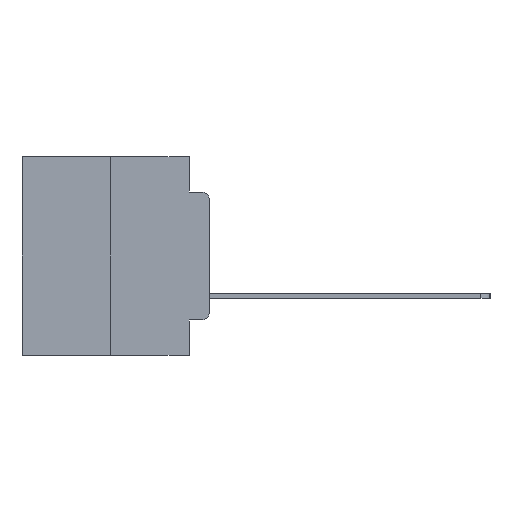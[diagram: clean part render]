
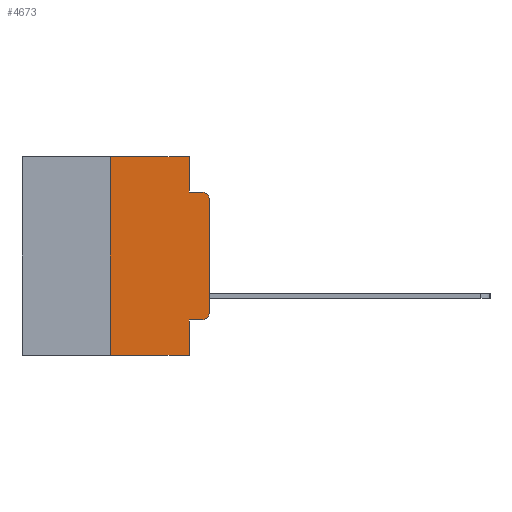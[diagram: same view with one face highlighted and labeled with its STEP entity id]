
A CAD part, left-side view. The second image highlights one B-rep face of the part: STEP entity #4673.
In plain terms, the highlighted planar face has unit normal (-1, 0, 0).
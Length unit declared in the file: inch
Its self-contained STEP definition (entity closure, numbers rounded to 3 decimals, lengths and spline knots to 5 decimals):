
#349 = VERTEX_POINT ( 'NONE', #19392 ) ;
#1485 = PLANE ( 'NONE',  #8360 ) ;
#1771 = VERTEX_POINT ( 'NONE', #16150 ) ;
#2369 = ORIENTED_EDGE ( 'NONE', *, *, #25255, .T. ) ;
#2727 = CARTESIAN_POINT ( 'NONE',  ( 0., 0.051, -0.4115 ) ) ;
#3296 = CARTESIAN_POINT ( 'NONE',  ( 0., 0.25, 0. ) ) ;
#3491 = ORIENTED_EDGE ( 'NONE', *, *, #5025, .F. ) ;
#3534 = ORIENTED_EDGE ( 'NONE', *, *, #21155, .T. ) ;
#3562 = ORIENTED_EDGE ( 'NONE', *, *, #26582, .F. ) ;
#3567 = EDGE_CURVE ( 'NONE', #19962, #5562, #17868, .T. ) ;
#3705 = DIRECTION ( 'NONE',  ( 1., 0., 0. ) ) ;
#3927 = ORIENTED_EDGE ( 'NONE', *, *, #9426, .F. ) ;
#3983 = ORIENTED_EDGE ( 'NONE', *, *, #23958, .T. ) ;
#4259 = ORIENTED_EDGE ( 'NONE', *, *, #13850, .T. ) ;
#4285 = ORIENTED_EDGE ( 'NONE', *, *, #6533, .F. ) ;
#4440 = ORIENTED_EDGE ( 'NONE', *, *, #3567, .F. ) ;
#4673 = ADVANCED_FACE ( 'NONE', ( #6286 ), #1485, .F. ) ;
#4761 = VERTEX_POINT ( 'NONE', #21596 ) ;
#4978 = CARTESIAN_POINT ( 'NONE',  ( 0., 0.02, -0.1085 ) ) ;
#5025 = EDGE_CURVE ( 'NONE', #25647, #19962, #12076, .T. ) ;
#5562 = VERTEX_POINT ( 'NONE', #14230 ) ;
#5737 = CARTESIAN_POINT ( 'NONE',  ( 0., 0., -0.3915 ) ) ;
#5856 = DIRECTION ( 'NONE',  ( 0., 0., -1. ) ) ;
#6286 = FACE_OUTER_BOUND ( 'NONE', #25017, .T. ) ;
#6459 = ORIENTED_EDGE ( 'NONE', *, *, #15336, .T. ) ;
#6533 = EDGE_CURVE ( 'NONE', #5562, #349, #7517, .T. ) ;
#6743 = DIRECTION ( 'NONE',  ( 0., -1., 0. ) ) ;
#6965 = VECTOR ( 'NONE', #24414, 39.37008 ) ;
#7105 = LINE ( 'NONE', #12990, #23252 ) ;
#7225 = DIRECTION ( 'NONE',  ( 0., 0., -1. ) ) ;
#7517 = LINE ( 'NONE', #12367, #17675 ) ;
#7937 = DIRECTION ( 'NONE',  ( -1., 0., 0. ) ) ;
#8360 = AXIS2_PLACEMENT_3D ( 'NONE', #20780, #3705, #18849 ) ;
#8370 = CARTESIAN_POINT ( 'NONE',  ( 0., 0.25, 0. ) ) ;
#9426 = EDGE_CURVE ( 'NONE', #349, #21223, #22350, .T. ) ;
#11704 = CARTESIAN_POINT ( 'NONE',  ( 0., 0., 0. ) ) ;
#12076 = LINE ( 'NONE', #3296, #6965 ) ;
#12367 = CARTESIAN_POINT ( 'NONE',  ( 0., 0.051, 0. ) ) ;
#12893 = DIRECTION ( 'NONE',  ( 0., -1., 0. ) ) ;
#12990 = CARTESIAN_POINT ( 'NONE',  ( 0., 0.051, 0. ) ) ;
#13131 = CARTESIAN_POINT ( 'NONE',  ( 0., 0.473, 0. ) ) ;
#13288 = LINE ( 'NONE', #11704, #20127 ) ;
#13850 = EDGE_CURVE ( 'NONE', #26014, #21223, #23939, .T. ) ;
#14230 = CARTESIAN_POINT ( 'NONE',  ( 0., 0.051, 0. ) ) ;
#14301 = CARTESIAN_POINT ( 'NONE',  ( 0., 0.02, -0.0885 ) ) ;
#15212 = DIRECTION ( 'NONE',  ( 0., 0., -1. ) ) ;
#15336 = EDGE_CURVE ( 'NONE', #25549, #26014, #13288, .T. ) ;
#16150 = CARTESIAN_POINT ( 'NONE',  ( 0., 0.02, -0.4115 ) ) ;
#16336 = VECTOR ( 'NONE', #6743, 39.37008 ) ;
#17388 = VECTOR ( 'NONE', #22041, 39.37008 ) ;
#17675 = VECTOR ( 'NONE', #5856, 39.37008 ) ;
#17868 = LINE ( 'NONE', #13131, #23221 ) ;
#18249 = CARTESIAN_POINT ( 'NONE',  ( 0., 0.473, -0.5 ) ) ;
#18409 = VERTEX_POINT ( 'NONE', #27358 ) ;
#18849 = DIRECTION ( 'NONE',  ( 0., 0., -1. ) ) ;
#19028 = CIRCLE ( 'NONE', #25271, 0.02 ) ;
#19392 = CARTESIAN_POINT ( 'NONE',  ( 0., 0.051, -0.0885 ) ) ;
#19962 = VERTEX_POINT ( 'NONE', #8370 ) ;
#19978 = DIRECTION ( 'NONE',  ( -1., 0., 0. ) ) ;
#20127 = VECTOR ( 'NONE', #26059, 39.37008 ) ;
#20250 = DIRECTION ( 'NONE',  ( 0., -1., 0. ) ) ;
#20681 = CARTESIAN_POINT ( 'NONE',  ( 0., 0.02, -0.3915 ) ) ;
#20780 = CARTESIAN_POINT ( 'NONE',  ( 0., 0.473, 0. ) ) ;
#20939 = CARTESIAN_POINT ( 'NONE',  ( 0., 0.25, -0.5 ) ) ;
#21155 = EDGE_CURVE ( 'NONE', #25647, #4761, #23820, .T. ) ;
#21223 = VERTEX_POINT ( 'NONE', #14301 ) ;
#21596 = CARTESIAN_POINT ( 'NONE',  ( 0., 0.051, -0.5 ) ) ;
#21989 = VECTOR ( 'NONE', #20250, 39.37008 ) ;
#22041 = DIRECTION ( 'NONE',  ( 0., -1., 0. ) ) ;
#22350 = LINE ( 'NONE', #25453, #16336 ) ;
#22724 = DIRECTION ( 'NONE',  ( 0., 0., -1. ) ) ;
#22760 = LINE ( 'NONE', #2727, #17388 ) ;
#23221 = VECTOR ( 'NONE', #12893, 39.37008 ) ;
#23252 = VECTOR ( 'NONE', #15212, 39.37008 ) ;
#23806 = CARTESIAN_POINT ( 'NONE',  ( 0., 0., -0.1085 ) ) ;
#23820 = LINE ( 'NONE', #18249, #21989 ) ;
#23939 = CIRCLE ( 'NONE', #24329, 0.02 ) ;
#23958 = EDGE_CURVE ( 'NONE', #1771, #25549, #19028, .T. ) ;
#24329 = AXIS2_PLACEMENT_3D ( 'NONE', #4978, #19978, #7225 ) ;
#24414 = DIRECTION ( 'NONE',  ( 0., 0., 1. ) ) ;
#25017 = EDGE_LOOP ( 'NONE', ( #6459, #4259, #3927, #4285, #4440, #3491, #3534, #3562, #2369, #3983 ) ) ;
#25255 = EDGE_CURVE ( 'NONE', #18409, #1771, #22760, .T. ) ;
#25271 = AXIS2_PLACEMENT_3D ( 'NONE', #20681, #7937, #22724 ) ;
#25453 = CARTESIAN_POINT ( 'NONE',  ( 0., 0.051, -0.0885 ) ) ;
#25549 = VERTEX_POINT ( 'NONE', #5737 ) ;
#25647 = VERTEX_POINT ( 'NONE', #20939 ) ;
#26014 = VERTEX_POINT ( 'NONE', #23806 ) ;
#26059 = DIRECTION ( 'NONE',  ( 0., 0., 1. ) ) ;
#26582 = EDGE_CURVE ( 'NONE', #18409, #4761, #7105, .T. ) ;
#27358 = CARTESIAN_POINT ( 'NONE',  ( 0., 0.051, -0.4115 ) ) ;
